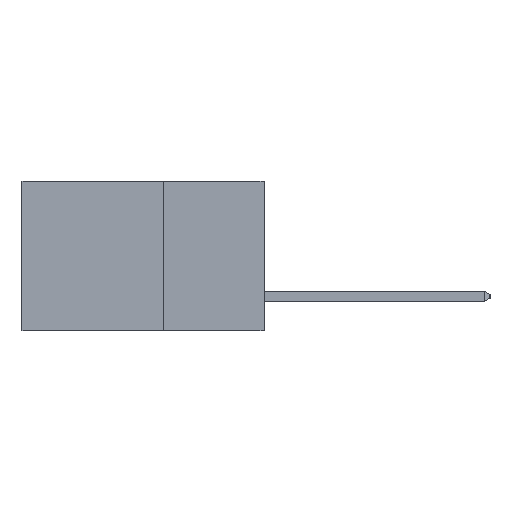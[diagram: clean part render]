
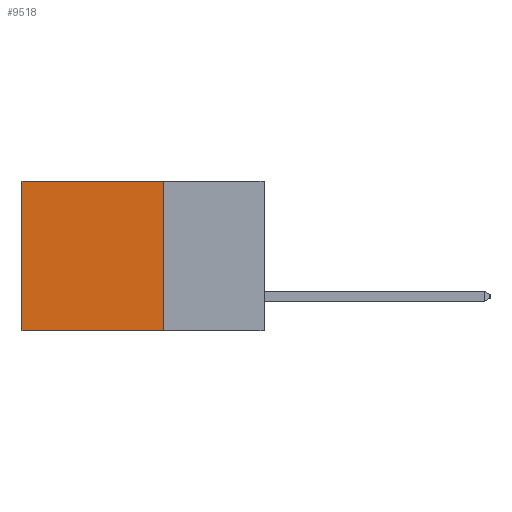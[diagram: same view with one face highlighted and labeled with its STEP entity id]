
A CAD part, left-side view. The second image highlights one B-rep face of the part: STEP entity #9518.
In plain terms, the highlighted planar face has unit normal (-1, 0, 0).
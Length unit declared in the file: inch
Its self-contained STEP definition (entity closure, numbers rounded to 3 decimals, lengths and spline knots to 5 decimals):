
#898 = ORIENTED_EDGE ( 'NONE', *, *, #2626, .F. ) ;
#921 = CARTESIAN_POINT ( 'NONE',  ( 0.2615, 0.6, 0. ) ) ;
#1469 = CARTESIAN_POINT ( 'NONE',  ( 0.2615, 0.6, -0.37 ) ) ;
#1483 = DIRECTION ( 'NONE',  ( 0., 0., -1. ) ) ;
#1819 = LINE ( 'NONE', #3378, #9013 ) ;
#1985 = VERTEX_POINT ( 'NONE', #7834 ) ;
#2053 = VECTOR ( 'NONE', #9527, 39.37008 ) ;
#2108 = CARTESIAN_POINT ( 'NONE',  ( 0.2615, 0.25, -0.37 ) ) ;
#2626 = EDGE_CURVE ( 'NONE', #10754, #1985, #7183, .T. ) ;
#2910 = EDGE_LOOP ( 'NONE', ( #4546, #7132, #898, #3476 ) ) ;
#3078 = CARTESIAN_POINT ( 'NONE',  ( 0.2615, 0.25, 0. ) ) ;
#3292 = CARTESIAN_POINT ( 'NONE',  ( 0.2615, 0.6, -0.37 ) ) ;
#3378 = CARTESIAN_POINT ( 'NONE',  ( 0.2615, 0.25, -0.37 ) ) ;
#3476 = ORIENTED_EDGE ( 'NONE', *, *, #11152, .T. ) ;
#4546 = ORIENTED_EDGE ( 'NONE', *, *, #8770, .T. ) ;
#5095 = VECTOR ( 'NONE', #1483, 39.37008 ) ;
#5105 = DIRECTION ( 'NONE',  ( 1., 0., 0. ) ) ;
#5340 = AXIS2_PLACEMENT_3D ( 'NONE', #2108, #5105, #11251 ) ;
#6586 = CARTESIAN_POINT ( 'NONE',  ( 0.2615, 0.25, 0. ) ) ;
#6803 = VERTEX_POINT ( 'NONE', #921 ) ;
#7132 = ORIENTED_EDGE ( 'NONE', *, *, #9716, .F. ) ;
#7183 = LINE ( 'NONE', #9492, #2053 ) ;
#7533 = LINE ( 'NONE', #1469, #5095 ) ;
#7834 = CARTESIAN_POINT ( 'NONE',  ( 0.2615, 0.25, -0.37 ) ) ;
#8439 = VECTOR ( 'NONE', #9232, 39.37008 ) ;
#8442 = VERTEX_POINT ( 'NONE', #3292 ) ;
#8682 = PLANE ( 'NONE',  #5340 ) ;
#8770 = EDGE_CURVE ( 'NONE', #6803, #8442, #7533, .T. ) ;
#9013 = VECTOR ( 'NONE', #9835, 39.37008 ) ;
#9232 = DIRECTION ( 'NONE',  ( 0., 1., 0. ) ) ;
#9492 = CARTESIAN_POINT ( 'NONE',  ( 0.2615, 0.25, -0.37 ) ) ;
#9518 = ADVANCED_FACE ( 'NONE', ( #10872 ), #8682, .F. ) ;
#9527 = DIRECTION ( 'NONE',  ( 0., 0., -1. ) ) ;
#9716 = EDGE_CURVE ( 'NONE', #1985, #8442, #1819, .T. ) ;
#9835 = DIRECTION ( 'NONE',  ( 0., 1., 0. ) ) ;
#10718 = LINE ( 'NONE', #6586, #8439 ) ;
#10754 = VERTEX_POINT ( 'NONE', #3078 ) ;
#10872 = FACE_OUTER_BOUND ( 'NONE', #2910, .T. ) ;
#11152 = EDGE_CURVE ( 'NONE', #10754, #6803, #10718, .T. ) ;
#11251 = DIRECTION ( 'NONE',  ( 0., 0., -1. ) ) ;
